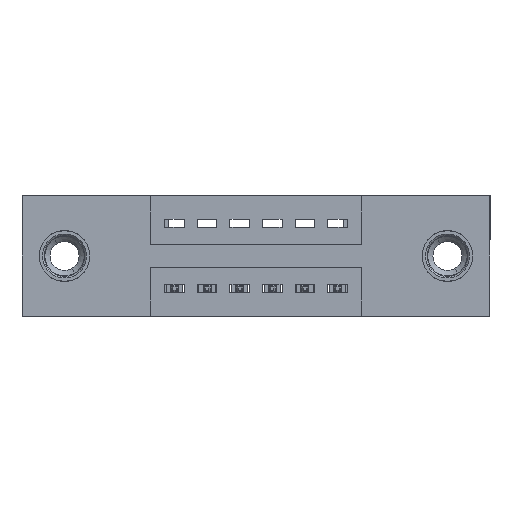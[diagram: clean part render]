
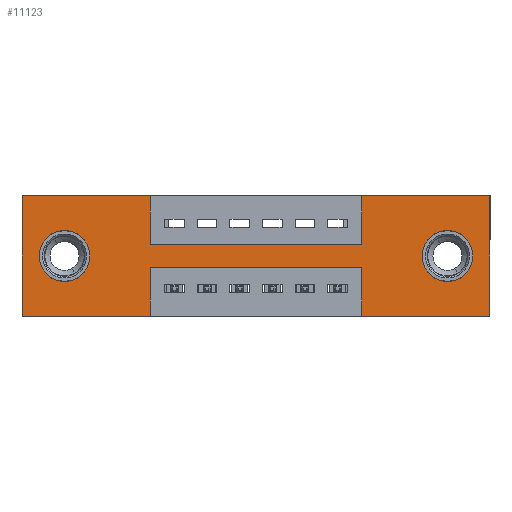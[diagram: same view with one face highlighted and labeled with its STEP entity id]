
A CAD part, front view. The second image highlights one B-rep face of the part: STEP entity #11123.
In plain terms, the highlighted planar face has unit normal (0, -1, 0).
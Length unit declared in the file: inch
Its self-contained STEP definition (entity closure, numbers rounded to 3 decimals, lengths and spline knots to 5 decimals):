
#3 = DIRECTION ( 'NONE',  ( 0., 0., 1. ) ) ;
#206 = AXIS2_PLACEMENT_3D ( 'NONE', #5691, #12383, #10215 ) ;
#350 = VECTOR ( 'NONE', #4480, 39.37008 ) ;
#454 = EDGE_CURVE ( 'NONE', #5633, #2894, #2123, .T. ) ;
#525 = CARTESIAN_POINT ( 'NONE',  ( 0., 0., -0.37 ) ) ;
#557 = CARTESIAN_POINT ( 'NONE',  ( 1.305, 0., -0.185 ) ) ;
#646 = EDGE_CURVE ( 'NONE', #6934, #5733, #1758, .T. ) ;
#1056 = VERTEX_POINT ( 'NONE', #10315 ) ;
#1105 = CARTESIAN_POINT ( 'NONE',  ( 0.3925, 0., 0. ) ) ;
#1215 = ORIENTED_EDGE ( 'NONE', *, *, #646, .F. ) ;
#1358 = ORIENTED_EDGE ( 'NONE', *, *, #12846, .F. ) ;
#1364 = CARTESIAN_POINT ( 'NONE',  ( 0., 0., -0.37 ) ) ;
#1574 = VECTOR ( 'NONE', #7927, 39.37008 ) ;
#1593 = CARTESIAN_POINT ( 'NONE',  ( 1.305, 0., -0.107 ) ) ;
#1695 = VERTEX_POINT ( 'NONE', #7187 ) ;
#1758 = LINE ( 'NONE', #10793, #12788 ) ;
#1762 = VECTOR ( 'NONE', #2714, 39.37008 ) ;
#1806 = ORIENTED_EDGE ( 'NONE', *, *, #10346, .F. ) ;
#1807 = CARTESIAN_POINT ( 'NONE',  ( 0., 0., 0. ) ) ;
#1823 = EDGE_CURVE ( 'NONE', #13552, #8075, #10318, .T. ) ;
#2096 = FACE_OUTER_BOUND ( 'NONE', #4423, .T. ) ;
#2123 = CIRCLE ( 'NONE', #10387, 0.078 ) ;
#2125 = VECTOR ( 'NONE', #3, 39.37008 ) ;
#2333 = DIRECTION ( 'NONE',  ( 0., -1., 0. ) ) ;
#2603 = EDGE_CURVE ( 'NONE', #13650, #1695, #12375, .T. ) ;
#2680 = AXIS2_PLACEMENT_3D ( 'NONE', #557, #12651, #7094 ) ;
#2714 = DIRECTION ( 'NONE',  ( -1., 0., 0. ) ) ;
#2725 = DIRECTION ( 'NONE',  ( 0., 1., 0. ) ) ;
#2775 = FACE_BOUND ( 'NONE', #12295, .T. ) ;
#2894 = VERTEX_POINT ( 'NONE', #3256 ) ;
#3256 = CARTESIAN_POINT ( 'NONE',  ( 0.13, 0., -0.107 ) ) ;
#3296 = CIRCLE ( 'NONE', #206, 0.078 ) ;
#3449 = LINE ( 'NONE', #7786, #350 ) ;
#3803 = CARTESIAN_POINT ( 'NONE',  ( 1.0425, 0., 0. ) ) ;
#4238 = EDGE_CURVE ( 'NONE', #13465, #6934, #14034, .T. ) ;
#4295 = VERTEX_POINT ( 'NONE', #5306 ) ;
#4334 = CARTESIAN_POINT ( 'NONE',  ( 0.13, 0., -0.263 ) ) ;
#4423 = EDGE_LOOP ( 'NONE', ( #1358, #1806, #5792, #6407, #6438, #7680, #12930, #11418, #9723, #1215, #4744, #7431 ) ) ;
#4480 = DIRECTION ( 'NONE',  ( 1., 0., 0. ) ) ;
#4482 = LINE ( 'NONE', #10617, #8076 ) ;
#4528 = VECTOR ( 'NONE', #6604, 39.37008 ) ;
#4744 = ORIENTED_EDGE ( 'NONE', *, *, #4238, .F. ) ;
#4840 = CARTESIAN_POINT ( 'NONE',  ( 1.435, 0., -0.37 ) ) ;
#4927 = ORIENTED_EDGE ( 'NONE', *, *, #11278, .T. ) ;
#5022 = DIRECTION ( 'NONE',  ( 0., 1., 0. ) ) ;
#5053 = EDGE_LOOP ( 'NONE', ( #5314, #4927 ) ) ;
#5158 = DIRECTION ( 'NONE',  ( 0., 0., -1. ) ) ;
#5175 = DIRECTION ( 'NONE',  ( 0., 0., 1. ) ) ;
#5306 = CARTESIAN_POINT ( 'NONE',  ( 0.3925, 0., -0.37 ) ) ;
#5314 = ORIENTED_EDGE ( 'NONE', *, *, #8920, .T. ) ;
#5633 = VERTEX_POINT ( 'NONE', #4334 ) ;
#5691 = CARTESIAN_POINT ( 'NONE',  ( 1.305, 0., -0.185 ) ) ;
#5733 = VERTEX_POINT ( 'NONE', #1105 ) ;
#5792 = ORIENTED_EDGE ( 'NONE', *, *, #1823, .F. ) ;
#5848 = CARTESIAN_POINT ( 'NONE',  ( 1.0425, 0., -0.37 ) ) ;
#5923 = LINE ( 'NONE', #525, #1762 ) ;
#5950 = VERTEX_POINT ( 'NONE', #7904 ) ;
#5992 = CARTESIAN_POINT ( 'NONE',  ( 0.3925, 0., -0.15 ) ) ;
#6114 = CARTESIAN_POINT ( 'NONE',  ( 0.13, 0., -0.185 ) ) ;
#6407 = ORIENTED_EDGE ( 'NONE', *, *, #8112, .F. ) ;
#6438 = ORIENTED_EDGE ( 'NONE', *, *, #10474, .F. ) ;
#6604 = DIRECTION ( 'NONE',  ( -1., 0., 0. ) ) ;
#6624 = LINE ( 'NONE', #10918, #2125 ) ;
#6934 = VERTEX_POINT ( 'NONE', #8507 ) ;
#7064 = LINE ( 'NONE', #8646, #12551 ) ;
#7094 = DIRECTION ( 'NONE',  ( 0., 0., -1. ) ) ;
#7113 = EDGE_CURVE ( 'NONE', #4295, #13465, #5923, .T. ) ;
#7187 = CARTESIAN_POINT ( 'NONE',  ( 1.0425, 0., -0.15 ) ) ;
#7348 = CARTESIAN_POINT ( 'NONE',  ( 0., 0., -0.37 ) ) ;
#7431 = ORIENTED_EDGE ( 'NONE', *, *, #7113, .F. ) ;
#7455 = CIRCLE ( 'NONE', #2680, 0.078 ) ;
#7493 = CARTESIAN_POINT ( 'NONE',  ( 0.3925, 0., -0.22 ) ) ;
#7585 = VECTOR ( 'NONE', #9142, 39.37008 ) ;
#7680 = ORIENTED_EDGE ( 'NONE', *, *, #12892, .F. ) ;
#7786 = CARTESIAN_POINT ( 'NONE',  ( 0., 0., 0. ) ) ;
#7863 = AXIS2_PLACEMENT_3D ( 'NONE', #11591, #5022, #10442 ) ;
#7904 = CARTESIAN_POINT ( 'NONE',  ( 1.305, 0., -0.263 ) ) ;
#7927 = DIRECTION ( 'NONE',  ( 0., 0., -1. ) ) ;
#7949 = FACE_BOUND ( 'NONE', #5053, .T. ) ;
#8075 = VERTEX_POINT ( 'NONE', #11890 ) ;
#8076 = VECTOR ( 'NONE', #5158, 39.37008 ) ;
#8112 = EDGE_CURVE ( 'NONE', #13159, #13552, #12572, .T. ) ;
#8447 = VECTOR ( 'NONE', #5175, 39.37008 ) ;
#8507 = CARTESIAN_POINT ( 'NONE',  ( 0., 0., 0. ) ) ;
#8574 = CARTESIAN_POINT ( 'NONE',  ( 1.0425, 0., -0.37 ) ) ;
#8576 = VECTOR ( 'NONE', #10510, 39.37008 ) ;
#8591 = DIRECTION ( 'NONE',  ( -1., 0., 0. ) ) ;
#8646 = CARTESIAN_POINT ( 'NONE',  ( 0.3925, 0., 0. ) ) ;
#8657 = VERTEX_POINT ( 'NONE', #7493 ) ;
#8918 = CARTESIAN_POINT ( 'NONE',  ( 0., 0., -0.37 ) ) ;
#8920 = EDGE_CURVE ( 'NONE', #11305, #5950, #3296, .T. ) ;
#8977 = VERTEX_POINT ( 'NONE', #3803 ) ;
#9142 = DIRECTION ( 'NONE',  ( 1., 0., 0. ) ) ;
#9303 = EDGE_CURVE ( 'NONE', #5733, #13650, #7064, .T. ) ;
#9723 = ORIENTED_EDGE ( 'NONE', *, *, #9303, .F. ) ;
#9758 = CARTESIAN_POINT ( 'NONE',  ( 0.3925, 0., -0.22 ) ) ;
#9799 = EDGE_CURVE ( 'NONE', #1695, #8977, #6624, .T. ) ;
#10029 = DIRECTION ( 'NONE',  ( 0., 0., -1. ) ) ;
#10215 = DIRECTION ( 'NONE',  ( 0., 0., -1. ) ) ;
#10315 = CARTESIAN_POINT ( 'NONE',  ( 1.435, 0., 0. ) ) ;
#10318 = LINE ( 'NONE', #8574, #8447 ) ;
#10346 = EDGE_CURVE ( 'NONE', #8075, #8657, #11896, .T. ) ;
#10387 = AXIS2_PLACEMENT_3D ( 'NONE', #6114, #2725, #10462 ) ;
#10442 = DIRECTION ( 'NONE',  ( 0., 0., 1. ) ) ;
#10462 = DIRECTION ( 'NONE',  ( 0., 0., 1. ) ) ;
#10474 = EDGE_CURVE ( 'NONE', #1056, #13159, #12251, .T. ) ;
#10510 = DIRECTION ( 'NONE',  ( 0., 0., 1. ) ) ;
#10617 = CARTESIAN_POINT ( 'NONE',  ( 0.3925, 0., -0.37 ) ) ;
#10793 = CARTESIAN_POINT ( 'NONE',  ( 0., 0., 0. ) ) ;
#10918 = CARTESIAN_POINT ( 'NONE',  ( 1.0425, 0., 0. ) ) ;
#11123 = ADVANCED_FACE ( 'NONE', ( #7949, #2775, #2096 ), #12279, .T. ) ;
#11257 = ORIENTED_EDGE ( 'NONE', *, *, #11678, .T. ) ;
#11278 = EDGE_CURVE ( 'NONE', #5950, #11305, #7455, .T. ) ;
#11305 = VERTEX_POINT ( 'NONE', #1593 ) ;
#11418 = ORIENTED_EDGE ( 'NONE', *, *, #2603, .F. ) ;
#11578 = CARTESIAN_POINT ( 'NONE',  ( 0.3925, 0., -0.15 ) ) ;
#11591 = CARTESIAN_POINT ( 'NONE',  ( 0.13, 0., -0.185 ) ) ;
#11678 = EDGE_CURVE ( 'NONE', #2894, #5633, #11718, .T. ) ;
#11718 = CIRCLE ( 'NONE', #7863, 0.078 ) ;
#11888 = DIRECTION ( 'NONE',  ( 1., 0., 0. ) ) ;
#11890 = CARTESIAN_POINT ( 'NONE',  ( 1.0425, 0., -0.22 ) ) ;
#11896 = LINE ( 'NONE', #9758, #4528 ) ;
#12251 = LINE ( 'NONE', #13425, #1574 ) ;
#12279 = PLANE ( 'NONE',  #12818 ) ;
#12295 = EDGE_LOOP ( 'NONE', ( #11257, #13828 ) ) ;
#12375 = LINE ( 'NONE', #5992, #7585 ) ;
#12383 = DIRECTION ( 'NONE',  ( 0., 1., 0. ) ) ;
#12551 = VECTOR ( 'NONE', #14138, 39.37008 ) ;
#12572 = LINE ( 'NONE', #7348, #13939 ) ;
#12651 = DIRECTION ( 'NONE',  ( 0., 1., 0. ) ) ;
#12788 = VECTOR ( 'NONE', #11888, 39.37008 ) ;
#12818 = AXIS2_PLACEMENT_3D ( 'NONE', #1364, #2333, #10029 ) ;
#12846 = EDGE_CURVE ( 'NONE', #8657, #4295, #4482, .T. ) ;
#12892 = EDGE_CURVE ( 'NONE', #8977, #1056, #3449, .T. ) ;
#12930 = ORIENTED_EDGE ( 'NONE', *, *, #9799, .F. ) ;
#13159 = VERTEX_POINT ( 'NONE', #4840 ) ;
#13425 = CARTESIAN_POINT ( 'NONE',  ( 1.435, 0., 0. ) ) ;
#13465 = VERTEX_POINT ( 'NONE', #8918 ) ;
#13552 = VERTEX_POINT ( 'NONE', #5848 ) ;
#13650 = VERTEX_POINT ( 'NONE', #11578 ) ;
#13828 = ORIENTED_EDGE ( 'NONE', *, *, #454, .T. ) ;
#13939 = VECTOR ( 'NONE', #8591, 39.37008 ) ;
#14034 = LINE ( 'NONE', #1807, #8576 ) ;
#14138 = DIRECTION ( 'NONE',  ( 0., 0., -1. ) ) ;
